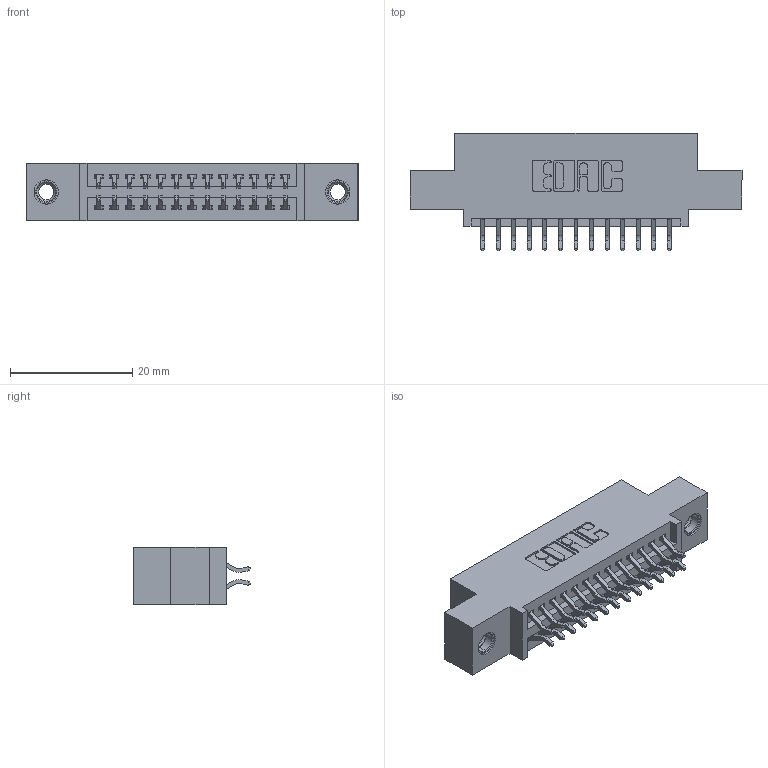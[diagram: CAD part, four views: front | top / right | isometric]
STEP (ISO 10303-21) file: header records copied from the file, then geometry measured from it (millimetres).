
FILE_DESCRIPTION (( 'STEP AP203' ), '1' );
FILE_NAME ('345-026-556-507.STEP', '2019-10-27T20:01:11', ( '' ), ( '' ), 'SwSTEP 2.0', 'SolidWorks 2016', '' );
FILE_SCHEMA (( 'CONFIG_CONTROL_DESIGN' ));
Length unit declared in the file: inch
Products named in the file (4): 345-292-001_556 Tail; 345-026-556-507; 345 Part_0.110 Offset - 0.156 Dia-TI; 345-250-001_345-250-005-103
Assembly tree (29 placements, depth 2):
  345-026-556-507
    345 Part_0.110 Offset - 0.156 Dia-TI
    345-292-001_556 Tail  x26
    345-250-001_345-250-005-103  x2
Bounding box: 54.23 x 19.24 x 9.4 mm (x, y, z)
Volume: 4910.8 mm3; surface area: 6795.2 mm2
Topology: 29 solids, 29 shells, 1646 faces, 4831 edges, 3178 vertices
Faces by surface type: plane 1078, cylinder 552, cone 12, torus 4
Entity records: 15642 total; most frequent: CARTESIAN_POINT 2647, ORIENTED_EDGE 2562, DIRECTION 2383, EDGE_CURVE 1281, LINE 1069, VECTOR 1069, VERTEX_POINT 848, AXIS2_PLACEMENT_3D 657
